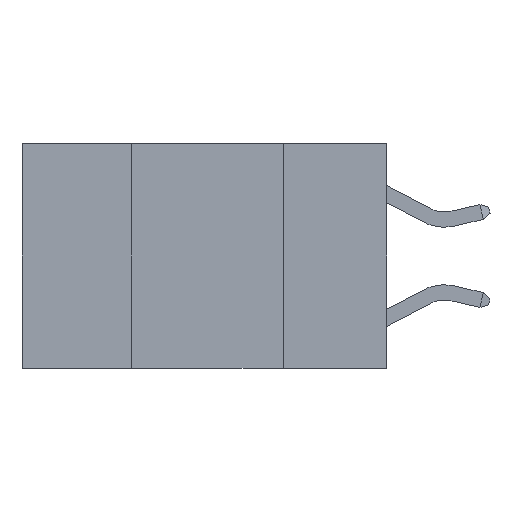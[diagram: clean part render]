
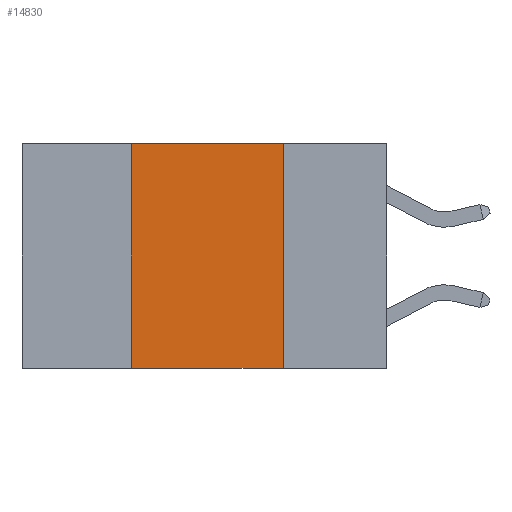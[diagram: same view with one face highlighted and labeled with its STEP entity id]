
A CAD part, left-side view. The second image highlights one B-rep face of the part: STEP entity #14830.
In plain terms, the highlighted planar face has unit normal (-1, 0, 0).
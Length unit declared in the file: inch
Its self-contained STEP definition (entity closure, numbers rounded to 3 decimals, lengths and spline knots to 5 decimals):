
#665 = VERTEX_POINT ( 'NONE', #23894 ) ;
#1204 = FACE_OUTER_BOUND ( 'NONE', #6330, .T. ) ;
#1843 = VECTOR ( 'NONE', #11413, 39.37008 ) ;
#1949 = EDGE_CURVE ( 'NONE', #19878, #3899, #11877, .T. ) ;
#2296 = CARTESIAN_POINT ( 'NONE',  ( 0., 0.6, 0. ) ) ;
#2523 = LINE ( 'NONE', #17623, #1843 ) ;
#2831 = EDGE_CURVE ( 'NONE', #665, #13075, #8938, .T. ) ;
#3172 = AXIS2_PLACEMENT_3D ( 'NONE', #2296, #21221, #8645 ) ;
#3899 = VERTEX_POINT ( 'NONE', #7886 ) ;
#5156 = DIRECTION ( 'NONE',  ( 0., -1., 0. ) ) ;
#6330 = EDGE_LOOP ( 'NONE', ( #22977, #8274, #14315, #17147 ) ) ;
#6887 = VECTOR ( 'NONE', #5156, 39.37008 ) ;
#7525 = CARTESIAN_POINT ( 'NONE',  ( 0., 0.42, 0. ) ) ;
#7886 = CARTESIAN_POINT ( 'NONE',  ( 0., 0.17, 0. ) ) ;
#8274 = ORIENTED_EDGE ( 'NONE', *, *, #1949, .F. ) ;
#8550 = PLANE ( 'NONE',  #3172 ) ;
#8645 = DIRECTION ( 'NONE',  ( 0., 0., -1. ) ) ;
#8824 = EDGE_CURVE ( 'NONE', #3899, #13075, #2523, .T. ) ;
#8938 = LINE ( 'NONE', #25340, #13891 ) ;
#11413 = DIRECTION ( 'NONE',  ( 0., 0., -1. ) ) ;
#11877 = LINE ( 'NONE', #21912, #6887 ) ;
#13075 = VERTEX_POINT ( 'NONE', #24936 ) ;
#13891 = VECTOR ( 'NONE', #23555, 39.37008 ) ;
#14315 = ORIENTED_EDGE ( 'NONE', *, *, #19192, .F. ) ;
#14830 = ADVANCED_FACE ( 'NONE', ( #1204 ), #8550, .F. ) ;
#17147 = ORIENTED_EDGE ( 'NONE', *, *, #2831, .T. ) ;
#17623 = CARTESIAN_POINT ( 'NONE',  ( 0., 0.17, 0. ) ) ;
#19192 = EDGE_CURVE ( 'NONE', #665, #19878, #22968, .T. ) ;
#19680 = CARTESIAN_POINT ( 'NONE',  ( 0., 0.42, 0. ) ) ;
#19878 = VERTEX_POINT ( 'NONE', #7525 ) ;
#21221 = DIRECTION ( 'NONE',  ( 1., 0., 0. ) ) ;
#21912 = CARTESIAN_POINT ( 'NONE',  ( 0., 0.6, 0. ) ) ;
#22305 = VECTOR ( 'NONE', #26071, 39.37008 ) ;
#22968 = LINE ( 'NONE', #19680, #22305 ) ;
#22977 = ORIENTED_EDGE ( 'NONE', *, *, #8824, .F. ) ;
#23555 = DIRECTION ( 'NONE',  ( 0., -1., 0. ) ) ;
#23894 = CARTESIAN_POINT ( 'NONE',  ( 0., 0.42, -0.37 ) ) ;
#24936 = CARTESIAN_POINT ( 'NONE',  ( 0., 0.17, -0.37 ) ) ;
#25340 = CARTESIAN_POINT ( 'NONE',  ( 0., 0.6, -0.37 ) ) ;
#26071 = DIRECTION ( 'NONE',  ( 0., 0., 1. ) ) ;
